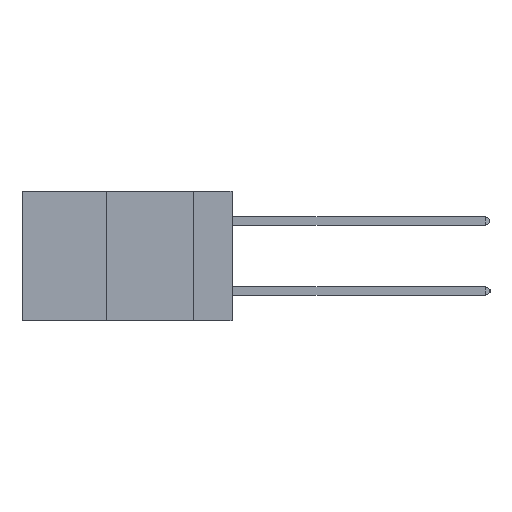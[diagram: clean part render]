
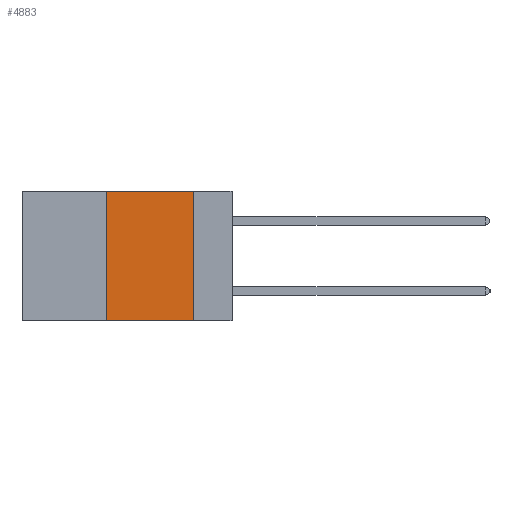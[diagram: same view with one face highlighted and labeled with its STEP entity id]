
A CAD part, left-side view. The second image highlights one B-rep face of the part: STEP entity #4883.
In plain terms, the highlighted planar face has unit normal (-1, 0, 0).
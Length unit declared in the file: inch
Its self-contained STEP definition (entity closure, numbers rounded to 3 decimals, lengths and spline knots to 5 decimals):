
#191 = CARTESIAN_POINT ( 'NONE',  ( 0., 0.6, 0. ) ) ;
#373 = FACE_OUTER_BOUND ( 'NONE', #3452, .T. ) ;
#515 = VECTOR ( 'NONE', #14034, 39.37008 ) ;
#758 = LINE ( 'NONE', #8434, #21644 ) ;
#3333 = CARTESIAN_POINT ( 'NONE',  ( 0., 0.36, 0. ) ) ;
#3452 = EDGE_LOOP ( 'NONE', ( #18772, #6562, #3833, #14434 ) ) ;
#3590 = CARTESIAN_POINT ( 'NONE',  ( 0., 0.6, -0.37 ) ) ;
#3833 = ORIENTED_EDGE ( 'NONE', *, *, #7846, .F. ) ;
#4013 = VECTOR ( 'NONE', #7176, 39.37008 ) ;
#4883 = ADVANCED_FACE ( 'NONE', ( #373 ), #7865, .F. ) ;
#5198 = VERTEX_POINT ( 'NONE', #21834 ) ;
#6445 = VECTOR ( 'NONE', #8468, 39.37008 ) ;
#6562 = ORIENTED_EDGE ( 'NONE', *, *, #19138, .F. ) ;
#7176 = DIRECTION ( 'NONE',  ( 0., -1., 0. ) ) ;
#7329 = EDGE_CURVE ( 'NONE', #13158, #21528, #21218, .T. ) ;
#7846 = EDGE_CURVE ( 'NONE', #13158, #11032, #19163, .T. ) ;
#7865 = PLANE ( 'NONE',  #10647 ) ;
#8434 = CARTESIAN_POINT ( 'NONE',  ( 0., 0.11, 0. ) ) ;
#8468 = DIRECTION ( 'NONE',  ( 0., 0., 1. ) ) ;
#9044 = CARTESIAN_POINT ( 'NONE',  ( 0., 0.36, 0. ) ) ;
#9884 = LINE ( 'NONE', #191, #515 ) ;
#10647 = AXIS2_PLACEMENT_3D ( 'NONE', #19417, #21049, #11242 ) ;
#11032 = VERTEX_POINT ( 'NONE', #9044 ) ;
#11242 = DIRECTION ( 'NONE',  ( 0., 0., -1. ) ) ;
#13158 = VERTEX_POINT ( 'NONE', #20698 ) ;
#14034 = DIRECTION ( 'NONE',  ( 0., -1., 0. ) ) ;
#14169 = CARTESIAN_POINT ( 'NONE',  ( 0., 0.11, -0.37 ) ) ;
#14434 = ORIENTED_EDGE ( 'NONE', *, *, #7329, .T. ) ;
#18337 = DIRECTION ( 'NONE',  ( 0., 0., -1. ) ) ;
#18772 = ORIENTED_EDGE ( 'NONE', *, *, #20227, .F. ) ;
#19138 = EDGE_CURVE ( 'NONE', #11032, #5198, #9884, .T. ) ;
#19163 = LINE ( 'NONE', #3333, #6445 ) ;
#19417 = CARTESIAN_POINT ( 'NONE',  ( 0., 0.6, 0. ) ) ;
#20227 = EDGE_CURVE ( 'NONE', #5198, #21528, #758, .T. ) ;
#20698 = CARTESIAN_POINT ( 'NONE',  ( 0., 0.36, -0.37 ) ) ;
#21049 = DIRECTION ( 'NONE',  ( 1., 0., 0. ) ) ;
#21218 = LINE ( 'NONE', #3590, #4013 ) ;
#21528 = VERTEX_POINT ( 'NONE', #14169 ) ;
#21644 = VECTOR ( 'NONE', #18337, 39.37008 ) ;
#21834 = CARTESIAN_POINT ( 'NONE',  ( 0., 0.11, 0. ) ) ;
